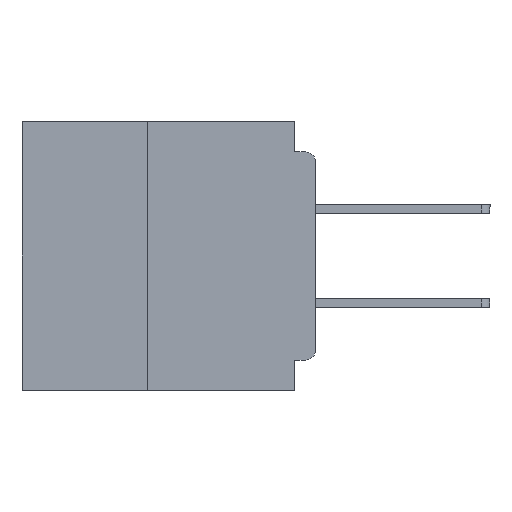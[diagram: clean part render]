
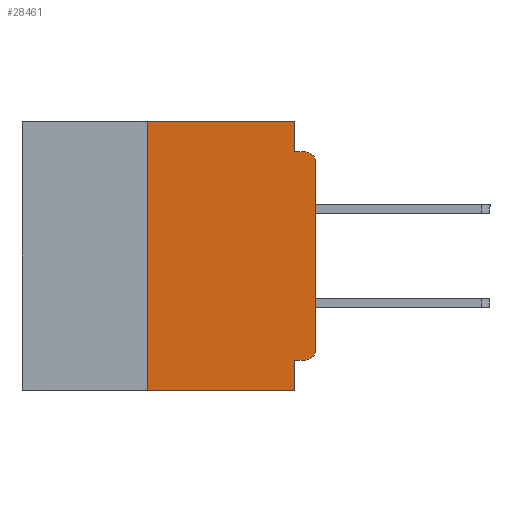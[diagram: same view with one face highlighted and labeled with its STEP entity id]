
A CAD part, left-side view. The second image highlights one B-rep face of the part: STEP entity #28461.
In plain terms, the highlighted planar face has unit normal (-1, 0, 0).
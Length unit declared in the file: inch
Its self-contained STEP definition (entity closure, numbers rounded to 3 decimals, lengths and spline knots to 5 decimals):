
#862 = VERTEX_POINT ( 'NONE', #47305 ) ;
#1179 = AXIS2_PLACEMENT_3D ( 'NONE', #22908, #15657, #41348 ) ;
#1652 = AXIS2_PLACEMENT_3D ( 'NONE', #5996, #31690, #9684 ) ;
#1964 = ORIENTED_EDGE ( 'NONE', *, *, #7775, .T. ) ;
#2319 = CARTESIAN_POINT ( 'NONE',  ( 0., 0.031, -0.4 ) ) ;
#2394 = EDGE_CURVE ( 'NONE', #6062, #9042, #38019, .T. ) ;
#2910 = EDGE_CURVE ( 'NONE', #26940, #9042, #6365, .T. ) ;
#2954 = VERTEX_POINT ( 'NONE', #31455 ) ;
#3098 = CARTESIAN_POINT ( 'NONE',  ( 0., 0.25, -0.4 ) ) ;
#3383 = ORIENTED_EDGE ( 'NONE', *, *, #2910, .T. ) ;
#4437 = CARTESIAN_POINT ( 'NONE',  ( 0., 0., -0.355 ) ) ;
#4902 = ORIENTED_EDGE ( 'NONE', *, *, #9820, .T. ) ;
#5976 = VERTEX_POINT ( 'NONE', #41381 ) ;
#5996 = CARTESIAN_POINT ( 'NONE',  ( 0., 0.015, -0.06 ) ) ;
#6062 = VERTEX_POINT ( 'NONE', #40203 ) ;
#6365 = LINE ( 'NONE', #32942, #14964 ) ;
#6622 = CARTESIAN_POINT ( 'NONE',  ( 0., 0.437, 0. ) ) ;
#7775 = EDGE_CURVE ( 'NONE', #8996, #46789, #34877, .T. ) ;
#8705 = VECTOR ( 'NONE', #44768, 39.37008 ) ;
#8995 = ORIENTED_EDGE ( 'NONE', *, *, #23146, .F. ) ;
#8996 = VERTEX_POINT ( 'NONE', #24052 ) ;
#9042 = VERTEX_POINT ( 'NONE', #2319 ) ;
#9684 = DIRECTION ( 'NONE',  ( 0., 0., -1. ) ) ;
#9820 = EDGE_CURVE ( 'NONE', #862, #8996, #39240, .T. ) ;
#9936 = VECTOR ( 'NONE', #37665, 39.37008 ) ;
#10139 = VECTOR ( 'NONE', #14409, 39.37008 ) ;
#10291 = DIRECTION ( 'NONE',  ( 0., -1., 0. ) ) ;
#10703 = CARTESIAN_POINT ( 'NONE',  ( 0., 0.25, -0.4 ) ) ;
#11867 = EDGE_LOOP ( 'NONE', ( #4902, #1964, #34204, #45066, #20399, #8995, #3383, #27839, #20526, #22087 ) ) ;
#11905 = DIRECTION ( 'NONE',  ( -1., 0., 0. ) ) ;
#13468 = DIRECTION ( 'NONE',  ( 0., -1., 0. ) ) ;
#13558 = VERTEX_POINT ( 'NONE', #35154 ) ;
#13613 = CARTESIAN_POINT ( 'NONE',  ( 0., 0.015, -0.045 ) ) ;
#14409 = DIRECTION ( 'NONE',  ( 0., 0., 1. ) ) ;
#14940 = EDGE_CURVE ( 'NONE', #13558, #24564, #43654, .T. ) ;
#14964 = VECTOR ( 'NONE', #32950, 39.37008 ) ;
#15657 = DIRECTION ( 'NONE',  ( 1., 0., 0. ) ) ;
#17803 = VECTOR ( 'NONE', #13468, 39.37008 ) ;
#18449 = EDGE_CURVE ( 'NONE', #5976, #862, #26635, .T. ) ;
#19910 = LINE ( 'NONE', #10703, #10139 ) ;
#20081 = DIRECTION ( 'NONE',  ( 0., 0., -1. ) ) ;
#20399 = ORIENTED_EDGE ( 'NONE', *, *, #14940, .F. ) ;
#20526 = ORIENTED_EDGE ( 'NONE', *, *, #23295, .F. ) ;
#21006 = EDGE_CURVE ( 'NONE', #2954, #46789, #35076, .T. ) ;
#22087 = ORIENTED_EDGE ( 'NONE', *, *, #18449, .T. ) ;
#22908 = CARTESIAN_POINT ( 'NONE',  ( 0., 0.437, 0. ) ) ;
#23146 = EDGE_CURVE ( 'NONE', #26940, #13558, #19910, .T. ) ;
#23295 = EDGE_CURVE ( 'NONE', #5976, #6062, #41147, .T. ) ;
#24052 = CARTESIAN_POINT ( 'NONE',  ( 0., 0., -0.06 ) ) ;
#24564 = VERTEX_POINT ( 'NONE', #31249 ) ;
#26222 = LINE ( 'NONE', #42089, #35990 ) ;
#26635 = CIRCLE ( 'NONE', #41054, 0.015 ) ;
#26940 = VERTEX_POINT ( 'NONE', #3098 ) ;
#27839 = ORIENTED_EDGE ( 'NONE', *, *, #2394, .F. ) ;
#28461 = ADVANCED_FACE ( 'NONE', ( #31475 ), #30275, .F. ) ;
#30275 = PLANE ( 'NONE',  #1179 ) ;
#31249 = CARTESIAN_POINT ( 'NONE',  ( 0., 0.031, 0. ) ) ;
#31389 = VECTOR ( 'NONE', #41204, 39.37008 ) ;
#31455 = CARTESIAN_POINT ( 'NONE',  ( 0., 0.031, -0.045 ) ) ;
#31475 = FACE_OUTER_BOUND ( 'NONE', #11867, .T. ) ;
#31690 = DIRECTION ( 'NONE',  ( -1., 0., 0. ) ) ;
#32942 = CARTESIAN_POINT ( 'NONE',  ( 0., 0.437, -0.4 ) ) ;
#32950 = DIRECTION ( 'NONE',  ( 0., -1., 0. ) ) ;
#33944 = CARTESIAN_POINT ( 'NONE',  ( 0., 0.015, -0.34 ) ) ;
#33948 = VECTOR ( 'NONE', #10291, 39.37008 ) ;
#33976 = CARTESIAN_POINT ( 'NONE',  ( 0., 0., 0. ) ) ;
#34204 = ORIENTED_EDGE ( 'NONE', *, *, #21006, .F. ) ;
#34877 = CIRCLE ( 'NONE', #1652, 0.015 ) ;
#35076 = LINE ( 'NONE', #46340, #17803 ) ;
#35154 = CARTESIAN_POINT ( 'NONE',  ( 0., 0.25, 0. ) ) ;
#35990 = VECTOR ( 'NONE', #20081, 39.37008 ) ;
#37629 = DIRECTION ( 'NONE',  ( 0., 0., -1. ) ) ;
#37665 = DIRECTION ( 'NONE',  ( 0., 0., 1. ) ) ;
#38019 = LINE ( 'NONE', #44864, #8705 ) ;
#39240 = LINE ( 'NONE', #33976, #9936 ) ;
#40203 = CARTESIAN_POINT ( 'NONE',  ( 0., 0.031, -0.355 ) ) ;
#41054 = AXIS2_PLACEMENT_3D ( 'NONE', #33944, #11905, #37629 ) ;
#41147 = LINE ( 'NONE', #4437, #31389 ) ;
#41204 = DIRECTION ( 'NONE',  ( 0., 1., 0. ) ) ;
#41348 = DIRECTION ( 'NONE',  ( 0., 0., -1. ) ) ;
#41381 = CARTESIAN_POINT ( 'NONE',  ( 0., 0.015, -0.355 ) ) ;
#42089 = CARTESIAN_POINT ( 'NONE',  ( 0., 0.031, 0. ) ) ;
#43654 = LINE ( 'NONE', #6622, #33948 ) ;
#44768 = DIRECTION ( 'NONE',  ( 0., 0., -1. ) ) ;
#44864 = CARTESIAN_POINT ( 'NONE',  ( 0., 0.031, -0.4 ) ) ;
#45066 = ORIENTED_EDGE ( 'NONE', *, *, #47254, .F. ) ;
#46340 = CARTESIAN_POINT ( 'NONE',  ( 0., 0., -0.045 ) ) ;
#46789 = VERTEX_POINT ( 'NONE', #13613 ) ;
#47254 = EDGE_CURVE ( 'NONE', #24564, #2954, #26222, .T. ) ;
#47305 = CARTESIAN_POINT ( 'NONE',  ( 0., 0., -0.34 ) ) ;
